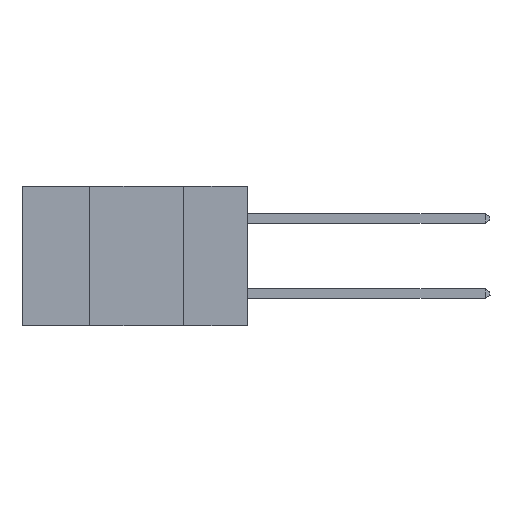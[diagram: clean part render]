
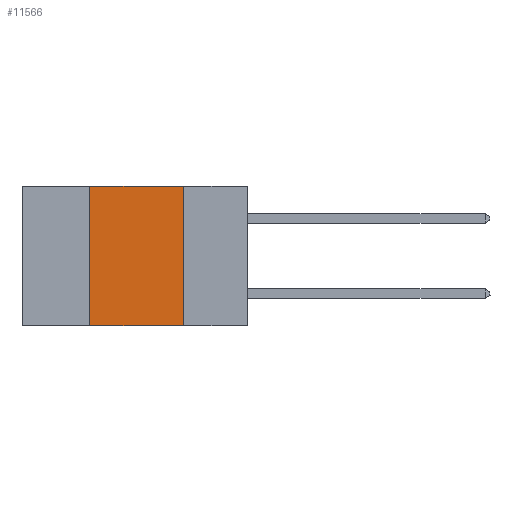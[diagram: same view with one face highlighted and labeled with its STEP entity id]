
A CAD part, left-side view. The second image highlights one B-rep face of the part: STEP entity #11566.
In plain terms, the highlighted planar face has unit normal (-1, 0, 0).
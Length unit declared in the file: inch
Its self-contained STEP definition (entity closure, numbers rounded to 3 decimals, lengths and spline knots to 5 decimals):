
#149 = DIRECTION ( 'NONE',  ( 0., 0., 1. ) ) ;
#339 = VERTEX_POINT ( 'NONE', #13760 ) ;
#438 = DIRECTION ( 'NONE',  ( 0., 0., -1. ) ) ;
#787 = LINE ( 'NONE', #1564, #9547 ) ;
#1564 = CARTESIAN_POINT ( 'NONE',  ( 0., 0.6, -0.37 ) ) ;
#2262 = EDGE_CURVE ( 'NONE', #9996, #339, #2517, .T. ) ;
#2268 = VERTEX_POINT ( 'NONE', #8105 ) ;
#2517 = LINE ( 'NONE', #6771, #12058 ) ;
#2974 = EDGE_CURVE ( 'NONE', #2268, #9996, #13640, .T. ) ;
#3101 = VECTOR ( 'NONE', #11864, 39.37008 ) ;
#3287 = ORIENTED_EDGE ( 'NONE', *, *, #2262, .F. ) ;
#3668 = CARTESIAN_POINT ( 'NONE',  ( 0., 0.42, -0.37 ) ) ;
#3671 = ORIENTED_EDGE ( 'NONE', *, *, #12431, .F. ) ;
#5343 = EDGE_CURVE ( 'NONE', #6681, #339, #787, .T. ) ;
#6508 = ORIENTED_EDGE ( 'NONE', *, *, #2974, .F. ) ;
#6681 = VERTEX_POINT ( 'NONE', #3668 ) ;
#6771 = CARTESIAN_POINT ( 'NONE',  ( 0., 0.17, 0. ) ) ;
#7896 = DIRECTION ( 'NONE',  ( 0., -1., 0. ) ) ;
#8105 = CARTESIAN_POINT ( 'NONE',  ( 0., 0.42, 0. ) ) ;
#8621 = AXIS2_PLACEMENT_3D ( 'NONE', #14246, #10340, #8991 ) ;
#8991 = DIRECTION ( 'NONE',  ( 0., 0., -1. ) ) ;
#9547 = VECTOR ( 'NONE', #7896, 39.37008 ) ;
#9996 = VERTEX_POINT ( 'NONE', #12886 ) ;
#10340 = DIRECTION ( 'NONE',  ( 1., 0., 0. ) ) ;
#11140 = FACE_OUTER_BOUND ( 'NONE', #16425, .T. ) ;
#11566 = ADVANCED_FACE ( 'NONE', ( #11140 ), #13794, .F. ) ;
#11778 = CARTESIAN_POINT ( 'NONE',  ( 0., 0.42, 0. ) ) ;
#11864 = DIRECTION ( 'NONE',  ( 0., -1., 0. ) ) ;
#12058 = VECTOR ( 'NONE', #438, 39.37008 ) ;
#12431 = EDGE_CURVE ( 'NONE', #6681, #2268, #13107, .T. ) ;
#12885 = ORIENTED_EDGE ( 'NONE', *, *, #5343, .T. ) ;
#12886 = CARTESIAN_POINT ( 'NONE',  ( 0., 0.17, 0. ) ) ;
#13107 = LINE ( 'NONE', #11778, #13304 ) ;
#13304 = VECTOR ( 'NONE', #149, 39.37008 ) ;
#13640 = LINE ( 'NONE', #14554, #3101 ) ;
#13760 = CARTESIAN_POINT ( 'NONE',  ( 0., 0.17, -0.37 ) ) ;
#13794 = PLANE ( 'NONE',  #8621 ) ;
#14246 = CARTESIAN_POINT ( 'NONE',  ( 0., 0.6, 0. ) ) ;
#14554 = CARTESIAN_POINT ( 'NONE',  ( 0., 0.6, 0. ) ) ;
#16425 = EDGE_LOOP ( 'NONE', ( #3287, #6508, #3671, #12885 ) ) ;
